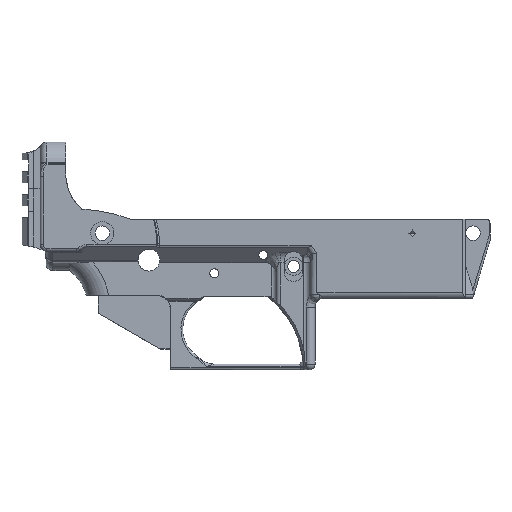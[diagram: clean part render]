
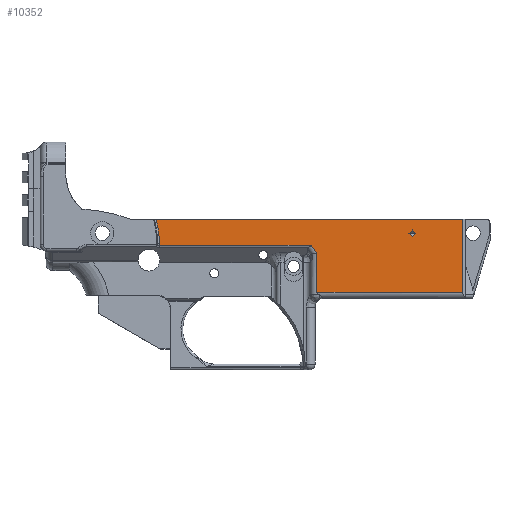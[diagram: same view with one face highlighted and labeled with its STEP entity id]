
A CAD part, left-side view. The second image highlights one B-rep face of the part: STEP entity #10352.
In plain terms, the highlighted planar face has unit normal (-1, 0, 0).
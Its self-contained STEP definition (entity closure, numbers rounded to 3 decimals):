
#201=FACE_BOUND('',#1253,.T.);
#240=ELLIPSE('',#11068,48.772,41.553);
#361=PLANE('',#11080);
#645=FACE_OUTER_BOUND('',#1252,.T.);
#1252=EDGE_LOOP('',(#7380,#7381,#7382,#7383,#7384,#7385,#7386,#7387));
#1253=EDGE_LOOP('',(#7388,#7389,#7390,#7391));
#2203=B_SPLINE_CURVE_WITH_KNOTS('',3,(#15914,#15915,#15916,#15917),
 .UNSPECIFIED.,.F.,.F.,(4,4),(-0.084,0.),
 .UNSPECIFIED.);
#2538=LINE('',#14539,#3340);
#2760=LINE('',#16094,#3562);
#2764=LINE('',#16109,#3566);
#2765=LINE('',#16112,#3567);
#2766=LINE('',#16114,#3568);
#2767=LINE('',#16115,#3569);
#2768=LINE('',#16118,#3570);
#2769=LINE('',#16120,#3571);
#2770=LINE('',#16122,#3572);
#2771=LINE('',#16123,#3573);
#3340=VECTOR('',#11847,154.067);
#3562=VECTOR('',#12421,10.);
#3566=VECTOR('',#12431,10.);
#3567=VECTOR('',#12434,53.92);
#3568=VECTOR('',#12435,10.);
#3569=VECTOR('',#12436,34.547);
#3570=VECTOR('',#12437,10.);
#3571=VECTOR('',#12438,10.);
#3572=VECTOR('',#12439,10.);
#3573=VECTOR('',#12440,10.);
#4150=VERTEX_POINT('',#14537);
#4151=VERTEX_POINT('',#14538);
#4458=VERTEX_POINT('',#15787);
#4459=VERTEX_POINT('',#15900);
#4480=VERTEX_POINT('',#16085);
#4482=VERTEX_POINT('',#16093);
#4485=VERTEX_POINT('',#16111);
#4486=VERTEX_POINT('',#16113);
#4487=VERTEX_POINT('',#16116);
#4488=VERTEX_POINT('',#16117);
#4489=VERTEX_POINT('',#16119);
#4490=VERTEX_POINT('',#16121);
#5189=EDGE_CURVE('',#4150,#4151,#2538,.T.);
#5565=EDGE_CURVE('',#4458,#4150,#240,.T.);
#5567=EDGE_CURVE('',#4459,#4458,#2203,.T.);
#5591=EDGE_CURVE('',#4480,#4482,#2760,.T.);
#5597=EDGE_CURVE('',#4482,#4459,#2764,.T.);
#5598=EDGE_CURVE('',#4485,#4480,#2765,.T.);
#5599=EDGE_CURVE('',#4486,#4485,#2766,.T.);
#5600=EDGE_CURVE('',#4151,#4486,#2767,.T.);
#5601=EDGE_CURVE('',#4487,#4488,#2768,.T.);
#5602=EDGE_CURVE('',#4488,#4489,#2769,.T.);
#5603=EDGE_CURVE('',#4489,#4490,#2770,.T.);
#5604=EDGE_CURVE('',#4490,#4487,#2771,.T.);
#7380=ORIENTED_EDGE('',*,*,#5598,.F.);
#7381=ORIENTED_EDGE('',*,*,#5599,.F.);
#7382=ORIENTED_EDGE('',*,*,#5600,.F.);
#7383=ORIENTED_EDGE('',*,*,#5189,.F.);
#7384=ORIENTED_EDGE('',*,*,#5565,.F.);
#7385=ORIENTED_EDGE('',*,*,#5567,.F.);
#7386=ORIENTED_EDGE('',*,*,#5597,.F.);
#7387=ORIENTED_EDGE('',*,*,#5591,.F.);
#7388=ORIENTED_EDGE('',*,*,#5601,.T.);
#7389=ORIENTED_EDGE('',*,*,#5602,.T.);
#7390=ORIENTED_EDGE('',*,*,#5603,.T.);
#7391=ORIENTED_EDGE('',*,*,#5604,.T.);
#10352=ADVANCED_FACE('',(#645,#201),#361,.F.);
#11068=AXIS2_PLACEMENT_3D('',#15789,#12393,#12394);
#11080=AXIS2_PLACEMENT_3D('',#16110,#12432,#12433);
#11847=DIRECTION('',(0.,-1.,0.));
#12393=DIRECTION('center_axis',(-1.,0.,0.));
#12394=DIRECTION('ref_axis',(0.,0.179,-0.984));
#12421=DIRECTION('',(0.,0.577,0.816));
#12431=DIRECTION('',(0.,1.,0.));
#12432=DIRECTION('center_axis',(1.,0.,0.));
#12433=DIRECTION('ref_axis',(0.,1.,0.));
#12434=DIRECTION('',(0.,0.,1.));
#12435=DIRECTION('',(0.,1.,0.));
#12436=DIRECTION('',(0.,0.,-1.));
#12437=DIRECTION('',(0.,0.707,-0.707));
#12438=DIRECTION('',(0.,0.707,0.707));
#12439=DIRECTION('',(0.,-0.707,0.707));
#12440=DIRECTION('',(0.,-0.707,-0.707));
#14537=CARTESIAN_POINT('',(-18.567,14.676,-47.419));
#14538=CARTESIAN_POINT('',(-18.567,-119.209,-47.419));
#14539=CARTESIAN_POINT('',(-18.567,34.858,-47.419));
#15787=CARTESIAN_POINT('',(-18.567,13.248,-57.945));
#15789=CARTESIAN_POINT('Origin',(-18.567,55.012,-62.807));
#15900=CARTESIAN_POINT('',(-18.567,13.395,-58.763));
#15914=CARTESIAN_POINT('Ctrl Pts',(-18.567,13.395,-58.763));
#15915=CARTESIAN_POINT('Ctrl Pts',(-18.567,13.292,-58.502));
#15916=CARTESIAN_POINT('Ctrl Pts',(-18.567,13.237,-58.225));
#15917=CARTESIAN_POINT('Ctrl Pts',(-18.567,13.248,-57.945));
#16085=CARTESIAN_POINT('',(-18.567,-55.482,-62.313));
#16093=CARTESIAN_POINT('',(-18.567,-52.972,-58.763));
#16094=CARTESIAN_POINT('',(-18.567,-37.405,-36.748));
#16109=CARTESIAN_POINT('',(-18.567,59.659,-58.763));
#16110=CARTESIAN_POINT('Origin',(-18.567,52.634,-63.933));
#16111=CARTESIAN_POINT('',(-18.567,-55.482,-79.427));
#16112=CARTESIAN_POINT('',(-18.567,-55.482,-59.289));
#16113=CARTESIAN_POINT('',(-18.567,-119.209,-79.427));
#16114=CARTESIAN_POINT('',(-18.567,-37.862,-79.427));
#16115=CARTESIAN_POINT('',(-18.567,-119.209,-47.419));
#16116=CARTESIAN_POINT('',(-18.567,-98.496,-53.532));
#16117=CARTESIAN_POINT('',(-18.567,-97.095,-54.933));
#16118=CARTESIAN_POINT('',(-18.567,-58.113,-93.915));
#16119=CARTESIAN_POINT('',(-18.567,-95.694,-53.532));
#16120=CARTESIAN_POINT('',(-18.567,-61.913,-19.751));
#16121=CARTESIAN_POINT('',(-18.567,-97.095,-52.131));
#16122=CARTESIAN_POINT('',(-18.567,-56.012,-93.215));
#16123=CARTESIAN_POINT('',(-18.567,-62.614,-17.65));
